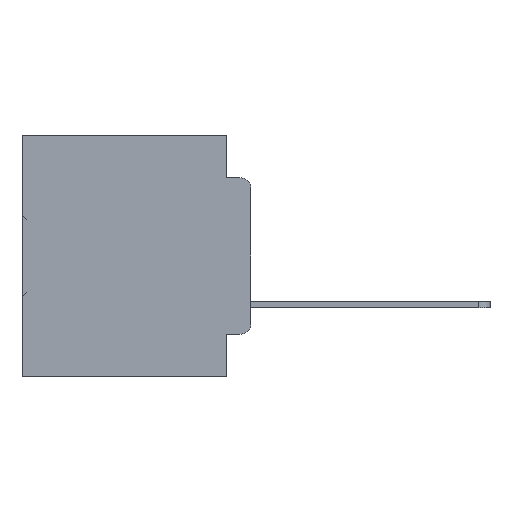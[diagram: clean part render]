
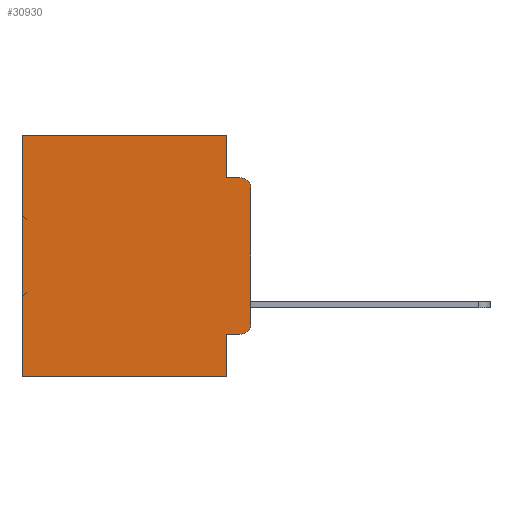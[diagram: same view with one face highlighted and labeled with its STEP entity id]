
A CAD part, left-side view. The second image highlights one B-rep face of the part: STEP entity #30930.
In plain terms, the highlighted planar face has unit normal (-1, 0, 0).
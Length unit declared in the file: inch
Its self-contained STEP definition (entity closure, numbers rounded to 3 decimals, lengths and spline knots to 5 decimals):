
#571 = CARTESIAN_POINT ( 'NONE',  ( 0.298, 0.051, 0. ) ) ;
#875 = ORIENTED_EDGE ( 'NONE', *, *, #12383, .T. ) ;
#1229 = LINE ( 'NONE', #6367, #31831 ) ;
#1614 = CARTESIAN_POINT ( 'NONE',  ( 0.298, 0.02, -0.0885 ) ) ;
#1690 = ORIENTED_EDGE ( 'NONE', *, *, #4995, .F. ) ;
#2334 = LINE ( 'NONE', #21125, #32495 ) ;
#4002 = DIRECTION ( 'NONE',  ( 0., 1., 0. ) ) ;
#4570 = VERTEX_POINT ( 'NONE', #7530 ) ;
#4948 = VERTEX_POINT ( 'NONE', #26621 ) ;
#4995 = EDGE_CURVE ( 'NONE', #8137, #13491, #1229, .T. ) ;
#5294 = CARTESIAN_POINT ( 'NONE',  ( 0.298, 0.051, -0.5 ) ) ;
#5383 = CARTESIAN_POINT ( 'NONE',  ( 0.298, 0.02, -0.4115 ) ) ;
#6317 = EDGE_CURVE ( 'NONE', #20497, #25173, #32196, .T. ) ;
#6367 = CARTESIAN_POINT ( 'NONE',  ( 0.298, 0.051, -0.0885 ) ) ;
#6827 = VERTEX_POINT ( 'NONE', #8499 ) ;
#7530 = CARTESIAN_POINT ( 'NONE',  ( 0.298, 0.473, 0. ) ) ;
#7580 = CARTESIAN_POINT ( 'NONE',  ( 0.298, 0., 0. ) ) ;
#7985 = LINE ( 'NONE', #36482, #19460 ) ;
#8137 = VERTEX_POINT ( 'NONE', #8689 ) ;
#8275 = EDGE_CURVE ( 'NONE', #20497, #13647, #2334, .T. ) ;
#8499 = CARTESIAN_POINT ( 'NONE',  ( 0.298, 0.473, -0.5 ) ) ;
#8636 = ORIENTED_EDGE ( 'NONE', *, *, #20420, .T. ) ;
#8689 = CARTESIAN_POINT ( 'NONE',  ( 0.298, 0.051, -0.0885 ) ) ;
#9500 = ORIENTED_EDGE ( 'NONE', *, *, #6317, .F. ) ;
#9564 = DIRECTION ( 'NONE',  ( 0., -1., 0. ) ) ;
#9597 = DIRECTION ( 'NONE',  ( 0., 1., 0. ) ) ;
#9633 = VECTOR ( 'NONE', #9597, 39.37008 ) ;
#10159 = DIRECTION ( 'NONE',  ( -1., 0., 0. ) ) ;
#10391 = DIRECTION ( 'NONE',  ( 0., 0., -1. ) ) ;
#10708 = EDGE_CURVE ( 'NONE', #4570, #6827, #34558, .T. ) ;
#11361 = FACE_OUTER_BOUND ( 'NONE', #35119, .T. ) ;
#12383 = EDGE_CURVE ( 'NONE', #34274, #13491, #26670, .T. ) ;
#13278 = CARTESIAN_POINT ( 'NONE',  ( 0.298, 0.02, -0.3915 ) ) ;
#13351 = ORIENTED_EDGE ( 'NONE', *, *, #21482, .T. ) ;
#13491 = VERTEX_POINT ( 'NONE', #1614 ) ;
#13647 = VERTEX_POINT ( 'NONE', #5383 ) ;
#14533 = ORIENTED_EDGE ( 'NONE', *, *, #29538, .F. ) ;
#15683 = CARTESIAN_POINT ( 'NONE',  ( 0.298, 0., 0. ) ) ;
#15809 = VECTOR ( 'NONE', #29902, 39.37008 ) ;
#16052 = DIRECTION ( 'NONE',  ( 0., 0., -1. ) ) ;
#16177 = DIRECTION ( 'NONE',  ( 0., 0., -1. ) ) ;
#16449 = CARTESIAN_POINT ( 'NONE',  ( 0.298, 0.051, -0.4115 ) ) ;
#16472 = DIRECTION ( 'NONE',  ( 0., 0., -1. ) ) ;
#17081 = LINE ( 'NONE', #15683, #34484 ) ;
#17228 = VERTEX_POINT ( 'NONE', #29146 ) ;
#17341 = AXIS2_PLACEMENT_3D ( 'NONE', #13278, #10159, #16052 ) ;
#17496 = LINE ( 'NONE', #571, #19323 ) ;
#18673 = CARTESIAN_POINT ( 'NONE',  ( 0.298, 0., -0.5 ) ) ;
#19248 = ORIENTED_EDGE ( 'NONE', *, *, #8275, .T. ) ;
#19274 = DIRECTION ( 'NONE',  ( -1., 0., 0. ) ) ;
#19323 = VECTOR ( 'NONE', #29593, 39.37008 ) ;
#19391 = ORIENTED_EDGE ( 'NONE', *, *, #28496, .F. ) ;
#19460 = VECTOR ( 'NONE', #4002, 39.37008 ) ;
#20420 = EDGE_CURVE ( 'NONE', #13647, #17228, #21402, .T. ) ;
#20497 = VERTEX_POINT ( 'NONE', #16449 ) ;
#21125 = CARTESIAN_POINT ( 'NONE',  ( 0.298, 0.051, -0.4115 ) ) ;
#21402 = CIRCLE ( 'NONE', #17341, 0.02 ) ;
#21482 = EDGE_CURVE ( 'NONE', #4948, #4570, #7985, .T. ) ;
#23279 = AXIS2_PLACEMENT_3D ( 'NONE', #28022, #19274, #16472 ) ;
#25173 = VERTEX_POINT ( 'NONE', #5294 ) ;
#26621 = CARTESIAN_POINT ( 'NONE',  ( 0.298, 0.051, 0. ) ) ;
#26670 = CIRCLE ( 'NONE', #23279, 0.02 ) ;
#26988 = AXIS2_PLACEMENT_3D ( 'NONE', #7580, #28099, #10391 ) ;
#27017 = DIRECTION ( 'NONE',  ( 0., -1., 0. ) ) ;
#28022 = CARTESIAN_POINT ( 'NONE',  ( 0.298, 0.02, -0.1085 ) ) ;
#28046 = EDGE_CURVE ( 'NONE', #34274, #17228, #17081, .T. ) ;
#28099 = DIRECTION ( 'NONE',  ( 1., 0., 0. ) ) ;
#28496 = EDGE_CURVE ( 'NONE', #4948, #8137, #17496, .T. ) ;
#29146 = CARTESIAN_POINT ( 'NONE',  ( 0.298, 0., -0.3915 ) ) ;
#29472 = ORIENTED_EDGE ( 'NONE', *, *, #28046, .F. ) ;
#29538 = EDGE_CURVE ( 'NONE', #25173, #6827, #32502, .T. ) ;
#29593 = DIRECTION ( 'NONE',  ( 0., 0., -1. ) ) ;
#29902 = DIRECTION ( 'NONE',  ( 0., 0., -1. ) ) ;
#30930 = ADVANCED_FACE ( 'NONE', ( #11361 ), #34826, .F. ) ;
#31831 = VECTOR ( 'NONE', #9564, 39.37008 ) ;
#31855 = ORIENTED_EDGE ( 'NONE', *, *, #10708, .T. ) ;
#32196 = LINE ( 'NONE', #34782, #34044 ) ;
#32495 = VECTOR ( 'NONE', #27017, 39.37008 ) ;
#32502 = LINE ( 'NONE', #18673, #9633 ) ;
#32838 = CARTESIAN_POINT ( 'NONE',  ( 0.298, 0.473, 0. ) ) ;
#34044 = VECTOR ( 'NONE', #37879, 39.37008 ) ;
#34274 = VERTEX_POINT ( 'NONE', #35725 ) ;
#34484 = VECTOR ( 'NONE', #16177, 39.37008 ) ;
#34558 = LINE ( 'NONE', #32838, #15809 ) ;
#34782 = CARTESIAN_POINT ( 'NONE',  ( 0.298, 0.051, 0. ) ) ;
#34826 = PLANE ( 'NONE',  #26988 ) ;
#35119 = EDGE_LOOP ( 'NONE', ( #29472, #875, #1690, #19391, #13351, #31855, #14533, #9500, #19248, #8636 ) ) ;
#35725 = CARTESIAN_POINT ( 'NONE',  ( 0.298, 0., -0.1085 ) ) ;
#36482 = CARTESIAN_POINT ( 'NONE',  ( 0.298, 0., 0. ) ) ;
#37879 = DIRECTION ( 'NONE',  ( 0., 0., -1. ) ) ;
